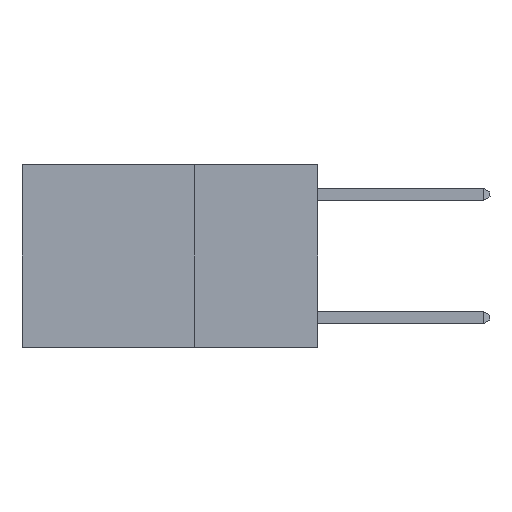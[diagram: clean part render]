
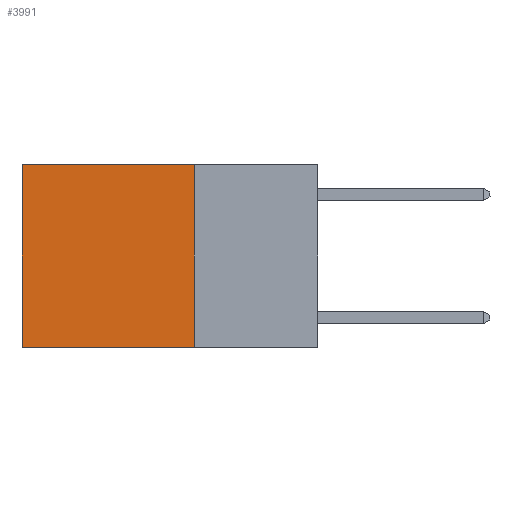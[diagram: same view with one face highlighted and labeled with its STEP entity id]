
A CAD part, left-side view. The second image highlights one B-rep face of the part: STEP entity #3991.
In plain terms, the highlighted planar face has unit normal (-1, 0, 0).
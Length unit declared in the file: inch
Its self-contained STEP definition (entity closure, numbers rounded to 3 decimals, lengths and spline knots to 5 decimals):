
#20 = CARTESIAN_POINT ( 'NONE',  ( 0.2625, 0.6, 0. ) ) ;
#93 = DIRECTION ( 'NONE',  ( 1., 0., 0. ) ) ;
#233 = CARTESIAN_POINT ( 'NONE',  ( 0.2625, 0.25, -0.37 ) ) ;
#335 = EDGE_CURVE ( 'NONE', #9390, #9761, #1647, .T. ) ;
#404 = PLANE ( 'NONE',  #3467 ) ;
#524 = DIRECTION ( 'NONE',  ( 0., 1., 0. ) ) ;
#1531 = FACE_OUTER_BOUND ( 'NONE', #5101, .T. ) ;
#1640 = VERTEX_POINT ( 'NONE', #9509 ) ;
#1647 = LINE ( 'NONE', #2115, #9919 ) ;
#1965 = ORIENTED_EDGE ( 'NONE', *, *, #6891, .F. ) ;
#2115 = CARTESIAN_POINT ( 'NONE',  ( 0.2625, 0.25, 0. ) ) ;
#2470 = VERTEX_POINT ( 'NONE', #3259 ) ;
#3259 = CARTESIAN_POINT ( 'NONE',  ( 0.2625, 0.25, -0.37 ) ) ;
#3381 = VECTOR ( 'NONE', #9647, 39.37008 ) ;
#3467 = AXIS2_PLACEMENT_3D ( 'NONE', #3935, #93, #8200 ) ;
#3935 = CARTESIAN_POINT ( 'NONE',  ( 0.2625, 0.25, 0. ) ) ;
#3991 = ADVANCED_FACE ( 'NONE', ( #1531 ), #404, .F. ) ;
#4821 = DIRECTION ( 'NONE',  ( 0., 0., -1. ) ) ;
#5101 = EDGE_LOOP ( 'NONE', ( #5988, #8149, #1965, #6231 ) ) ;
#5868 = CARTESIAN_POINT ( 'NONE',  ( 0.2625, 0.6, 0. ) ) ;
#5988 = ORIENTED_EDGE ( 'NONE', *, *, #8220, .T. ) ;
#6231 = ORIENTED_EDGE ( 'NONE', *, *, #335, .T. ) ;
#6401 = CARTESIAN_POINT ( 'NONE',  ( 0.2625, 0.25, 0. ) ) ;
#6653 = DIRECTION ( 'NONE',  ( 0., 1., 0. ) ) ;
#6891 = EDGE_CURVE ( 'NONE', #9390, #2470, #7916, .T. ) ;
#6961 = CARTESIAN_POINT ( 'NONE',  ( 0.2625, 0.25, 0. ) ) ;
#7916 = LINE ( 'NONE', #6401, #9773 ) ;
#8149 = ORIENTED_EDGE ( 'NONE', *, *, #8413, .F. ) ;
#8200 = DIRECTION ( 'NONE',  ( 0., 0., -1. ) ) ;
#8220 = EDGE_CURVE ( 'NONE', #9761, #1640, #9749, .T. ) ;
#8413 = EDGE_CURVE ( 'NONE', #2470, #1640, #10083, .T. ) ;
#9390 = VERTEX_POINT ( 'NONE', #6961 ) ;
#9509 = CARTESIAN_POINT ( 'NONE',  ( 0.2625, 0.6, -0.37 ) ) ;
#9626 = VECTOR ( 'NONE', #6653, 39.37008 ) ;
#9647 = DIRECTION ( 'NONE',  ( 0., 0., -1. ) ) ;
#9749 = LINE ( 'NONE', #20, #3381 ) ;
#9761 = VERTEX_POINT ( 'NONE', #5868 ) ;
#9773 = VECTOR ( 'NONE', #4821, 39.37008 ) ;
#9919 = VECTOR ( 'NONE', #524, 39.37008 ) ;
#10083 = LINE ( 'NONE', #233, #9626 ) ;
